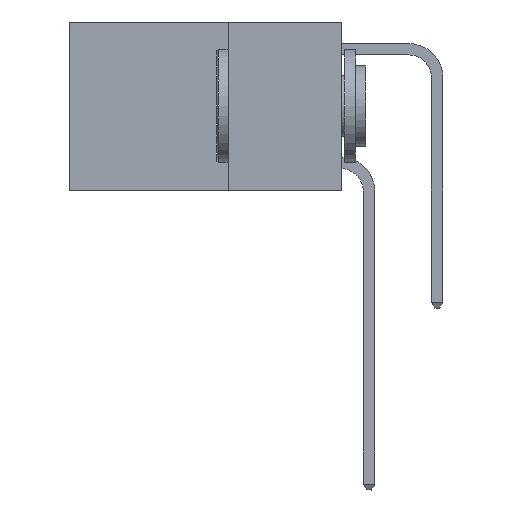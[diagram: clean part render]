
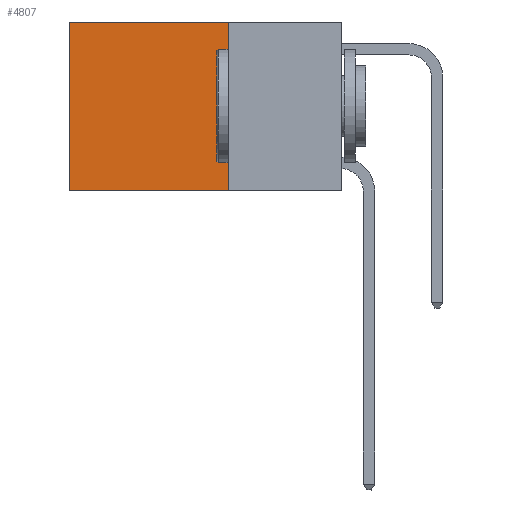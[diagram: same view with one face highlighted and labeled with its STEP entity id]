
A CAD part, left-side view. The second image highlights one B-rep face of the part: STEP entity #4807.
In plain terms, the highlighted planar face has unit normal (-1, 0, 0).
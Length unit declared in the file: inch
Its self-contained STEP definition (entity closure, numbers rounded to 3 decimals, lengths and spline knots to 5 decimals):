
#361 = VECTOR ( 'NONE', #12321, 39.37008 ) ;
#1393 = DIRECTION ( 'NONE',  ( 0., 0., -1. ) ) ;
#1682 = VECTOR ( 'NONE', #11326, 39.37008 ) ;
#1914 = EDGE_CURVE ( 'NONE', #10358, #6737, #9211, .T. ) ;
#2257 = VERTEX_POINT ( 'NONE', #20650 ) ;
#2890 = VERTEX_POINT ( 'NONE', #13592 ) ;
#4336 = ORIENTED_EDGE ( 'NONE', *, *, #8436, .F. ) ;
#4632 = CARTESIAN_POINT ( 'NONE',  ( 0.2625, 0.6, 0. ) ) ;
#4807 = ADVANCED_FACE ( 'NONE', ( #16897 ), #5391, .F. ) ;
#5207 = DIRECTION ( 'NONE',  ( 0., 0., -1. ) ) ;
#5391 = PLANE ( 'NONE',  #9784 ) ;
#6737 = VERTEX_POINT ( 'NONE', #9916 ) ;
#7308 = CARTESIAN_POINT ( 'NONE',  ( 0.2625, 0.25, 0. ) ) ;
#7395 = DIRECTION ( 'NONE',  ( 1., 0., 0. ) ) ;
#7514 = EDGE_CURVE ( 'NONE', #2890, #10358, #11627, .T. ) ;
#7535 = LINE ( 'NONE', #11140, #12221 ) ;
#8436 = EDGE_CURVE ( 'NONE', #2890, #2257, #7535, .T. ) ;
#9211 = LINE ( 'NONE', #23246, #19160 ) ;
#9784 = AXIS2_PLACEMENT_3D ( 'NONE', #7308, #7395, #21327 ) ;
#9916 = CARTESIAN_POINT ( 'NONE',  ( 0.2625, 0.6, -0.37 ) ) ;
#10253 = ORIENTED_EDGE ( 'NONE', *, *, #7514, .T. ) ;
#10317 = CARTESIAN_POINT ( 'NONE',  ( 0.2625, 0.25, 0. ) ) ;
#10358 = VERTEX_POINT ( 'NONE', #4632 ) ;
#11140 = CARTESIAN_POINT ( 'NONE',  ( 0.2625, 0.25, 0. ) ) ;
#11326 = DIRECTION ( 'NONE',  ( 0., 1., 0. ) ) ;
#11627 = LINE ( 'NONE', #10317, #361 ) ;
#12221 = VECTOR ( 'NONE', #5207, 39.37008 ) ;
#12321 = DIRECTION ( 'NONE',  ( 0., 1., 0. ) ) ;
#12373 = EDGE_CURVE ( 'NONE', #2257, #6737, #22282, .T. ) ;
#13592 = CARTESIAN_POINT ( 'NONE',  ( 0.2625, 0.25, 0. ) ) ;
#15868 = EDGE_LOOP ( 'NONE', ( #23759, #25652, #4336, #10253 ) ) ;
#16897 = FACE_OUTER_BOUND ( 'NONE', #15868, .T. ) ;
#19160 = VECTOR ( 'NONE', #1393, 39.37008 ) ;
#20650 = CARTESIAN_POINT ( 'NONE',  ( 0.2625, 0.25, -0.37 ) ) ;
#21327 = DIRECTION ( 'NONE',  ( 0., 0., -1. ) ) ;
#22282 = LINE ( 'NONE', #25181, #1682 ) ;
#23246 = CARTESIAN_POINT ( 'NONE',  ( 0.2625, 0.6, 0. ) ) ;
#23759 = ORIENTED_EDGE ( 'NONE', *, *, #1914, .T. ) ;
#25181 = CARTESIAN_POINT ( 'NONE',  ( 0.2625, 0.25, -0.37 ) ) ;
#25652 = ORIENTED_EDGE ( 'NONE', *, *, #12373, .F. ) ;
